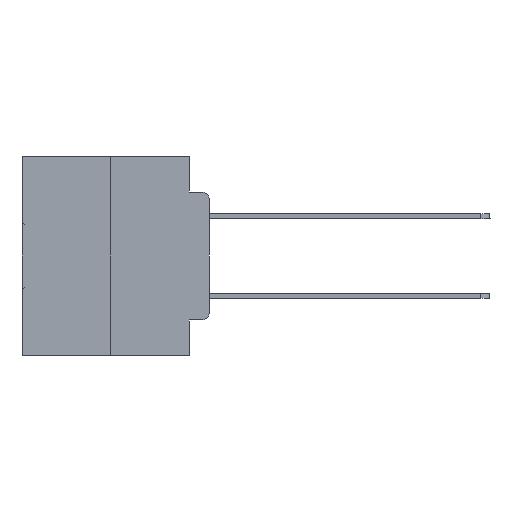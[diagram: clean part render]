
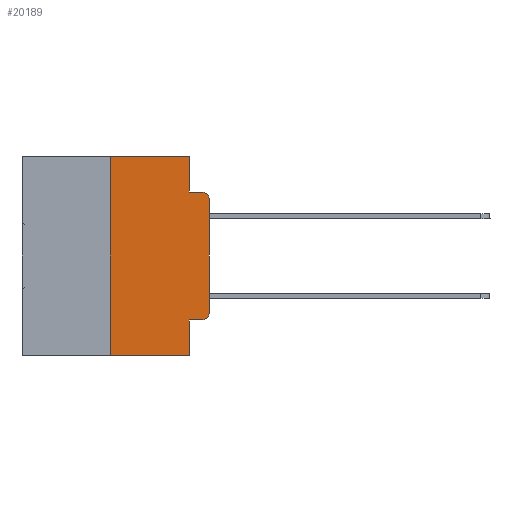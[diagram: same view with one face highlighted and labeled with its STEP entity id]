
A CAD part, left-side view. The second image highlights one B-rep face of the part: STEP entity #20189.
In plain terms, the highlighted planar face has unit normal (-1, 0, 0).
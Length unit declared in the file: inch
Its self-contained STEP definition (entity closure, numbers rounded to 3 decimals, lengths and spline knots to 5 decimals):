
#21 = EDGE_CURVE ( 'NONE', #10992, #4119, #4893, .T. ) ;
#157 = FACE_OUTER_BOUND ( 'NONE', #27811, .T. ) ;
#627 = EDGE_CURVE ( 'NONE', #30344, #17834, #30908, .T. ) ;
#1115 = DIRECTION ( 'NONE',  ( 0., 0., 1. ) ) ;
#1640 = LINE ( 'NONE', #12369, #16168 ) ;
#1830 = DIRECTION ( 'NONE',  ( -1., 0., 0. ) ) ;
#4119 = VERTEX_POINT ( 'NONE', #19429 ) ;
#4322 = VECTOR ( 'NONE', #1115, 39.37008 ) ;
#4497 = EDGE_CURVE ( 'NONE', #16200, #17834, #29449, .T. ) ;
#4893 = LINE ( 'NONE', #7351, #24763 ) ;
#5707 = ORIENTED_EDGE ( 'NONE', *, *, #21, .F. ) ;
#6244 = LINE ( 'NONE', #22634, #21636 ) ;
#6735 = CARTESIAN_POINT ( 'NONE',  ( 0., 0.051, -0.4115 ) ) ;
#6904 = DIRECTION ( 'NONE',  ( 0., -1., 0. ) ) ;
#7351 = CARTESIAN_POINT ( 'NONE',  ( 0., 0.473, 0. ) ) ;
#7398 = VERTEX_POINT ( 'NONE', #20386 ) ;
#7595 = VERTEX_POINT ( 'NONE', #31329 ) ;
#7841 = ORIENTED_EDGE ( 'NONE', *, *, #19334, .T. ) ;
#7988 = DIRECTION ( 'NONE',  ( 0., 0., -1. ) ) ;
#8205 = CARTESIAN_POINT ( 'NONE',  ( 0., 0.051, 0. ) ) ;
#8930 = CARTESIAN_POINT ( 'NONE',  ( 0., 0., -0.1085 ) ) ;
#10027 = DIRECTION ( 'NONE',  ( 0., -1., 0. ) ) ;
#10992 = VERTEX_POINT ( 'NONE', #23902 ) ;
#12167 = VECTOR ( 'NONE', #31198, 39.37008 ) ;
#12369 = CARTESIAN_POINT ( 'NONE',  ( 0., 0.473, -0.5 ) ) ;
#12485 = CARTESIAN_POINT ( 'NONE',  ( 0., 0.051, -0.4115 ) ) ;
#12622 = CARTESIAN_POINT ( 'NONE',  ( 0., 0.051, 0. ) ) ;
#12657 = DIRECTION ( 'NONE',  ( 0., 0., -1. ) ) ;
#14103 = CIRCLE ( 'NONE', #21765, 0.02 ) ;
#14610 = VERTEX_POINT ( 'NONE', #6735 ) ;
#14929 = CARTESIAN_POINT ( 'NONE',  ( 0., 0.051, -0.5 ) ) ;
#15437 = VECTOR ( 'NONE', #7988, 39.37008 ) ;
#15828 = LINE ( 'NONE', #8205, #15437 ) ;
#15901 = ORIENTED_EDGE ( 'NONE', *, *, #32395, .T. ) ;
#16168 = VECTOR ( 'NONE', #6904, 39.37008 ) ;
#16200 = VERTEX_POINT ( 'NONE', #26914 ) ;
#17142 = DIRECTION ( 'NONE',  ( 0., 0., 1. ) ) ;
#17507 = CARTESIAN_POINT ( 'NONE',  ( 0., 0.02, -0.0885 ) ) ;
#17512 = VECTOR ( 'NONE', #31790, 39.37008 ) ;
#17834 = VERTEX_POINT ( 'NONE', #17507 ) ;
#18859 = VECTOR ( 'NONE', #33964, 39.37008 ) ;
#19145 = EDGE_CURVE ( 'NONE', #14610, #24751, #33322, .T. ) ;
#19186 = LINE ( 'NONE', #12485, #12167 ) ;
#19246 = PLANE ( 'NONE',  #25090 ) ;
#19334 = EDGE_CURVE ( 'NONE', #7398, #30344, #24176, .T. ) ;
#19429 = CARTESIAN_POINT ( 'NONE',  ( 0., 0.051, 0. ) ) ;
#19983 = ORIENTED_EDGE ( 'NONE', *, *, #627, .T. ) ;
#20015 = ORIENTED_EDGE ( 'NONE', *, *, #24939, .T. ) ;
#20189 = ADVANCED_FACE ( 'NONE', ( #157 ), #19246, .F. ) ;
#20386 = CARTESIAN_POINT ( 'NONE',  ( 0., 0., -0.3915 ) ) ;
#20671 = ORIENTED_EDGE ( 'NONE', *, *, #30742, .F. ) ;
#21022 = VERTEX_POINT ( 'NONE', #25973 ) ;
#21636 = VECTOR ( 'NONE', #17142, 39.37008 ) ;
#21765 = AXIS2_PLACEMENT_3D ( 'NONE', #30863, #1830, #22782 ) ;
#21928 = ORIENTED_EDGE ( 'NONE', *, *, #4497, .F. ) ;
#22634 = CARTESIAN_POINT ( 'NONE',  ( 0., 0.25, 0. ) ) ;
#22782 = DIRECTION ( 'NONE',  ( 0., 0., -1. ) ) ;
#23088 = ORIENTED_EDGE ( 'NONE', *, *, #26561, .F. ) ;
#23142 = DIRECTION ( 'NONE',  ( -1., 0., 0. ) ) ;
#23608 = AXIS2_PLACEMENT_3D ( 'NONE', #28448, #23142, #12657 ) ;
#23902 = CARTESIAN_POINT ( 'NONE',  ( 0., 0.25, 0. ) ) ;
#24176 = LINE ( 'NONE', #24869, #4322 ) ;
#24551 = DIRECTION ( 'NONE',  ( 1., 0., 0. ) ) ;
#24751 = VERTEX_POINT ( 'NONE', #14929 ) ;
#24763 = VECTOR ( 'NONE', #10027, 39.37008 ) ;
#24869 = CARTESIAN_POINT ( 'NONE',  ( 0., 0., 0. ) ) ;
#24939 = EDGE_CURVE ( 'NONE', #14610, #21022, #19186, .T. ) ;
#25090 = AXIS2_PLACEMENT_3D ( 'NONE', #32549, #24551, #29836 ) ;
#25973 = CARTESIAN_POINT ( 'NONE',  ( 0., 0.02, -0.4115 ) ) ;
#26456 = CARTESIAN_POINT ( 'NONE',  ( 0., 0.051, -0.0885 ) ) ;
#26561 = EDGE_CURVE ( 'NONE', #7595, #10992, #6244, .T. ) ;
#26914 = CARTESIAN_POINT ( 'NONE',  ( 0., 0.051, -0.0885 ) ) ;
#27497 = EDGE_CURVE ( 'NONE', #7595, #24751, #1640, .T. ) ;
#27811 = EDGE_LOOP ( 'NONE', ( #7841, #19983, #21928, #20671, #5707, #23088, #30652, #33040, #20015, #15901 ) ) ;
#28448 = CARTESIAN_POINT ( 'NONE',  ( 0., 0.02, -0.1085 ) ) ;
#29449 = LINE ( 'NONE', #26456, #17512 ) ;
#29836 = DIRECTION ( 'NONE',  ( 0., 0., -1. ) ) ;
#30344 = VERTEX_POINT ( 'NONE', #8930 ) ;
#30652 = ORIENTED_EDGE ( 'NONE', *, *, #27497, .T. ) ;
#30742 = EDGE_CURVE ( 'NONE', #4119, #16200, #15828, .T. ) ;
#30863 = CARTESIAN_POINT ( 'NONE',  ( 0., 0.02, -0.3915 ) ) ;
#30908 = CIRCLE ( 'NONE', #23608, 0.02 ) ;
#31198 = DIRECTION ( 'NONE',  ( 0., -1., 0. ) ) ;
#31329 = CARTESIAN_POINT ( 'NONE',  ( 0., 0.25, -0.5 ) ) ;
#31790 = DIRECTION ( 'NONE',  ( 0., -1., 0. ) ) ;
#32395 = EDGE_CURVE ( 'NONE', #21022, #7398, #14103, .T. ) ;
#32549 = CARTESIAN_POINT ( 'NONE',  ( 0., 0.473, 0. ) ) ;
#33040 = ORIENTED_EDGE ( 'NONE', *, *, #19145, .F. ) ;
#33322 = LINE ( 'NONE', #12622, #18859 ) ;
#33964 = DIRECTION ( 'NONE',  ( 0., 0., -1. ) ) ;
